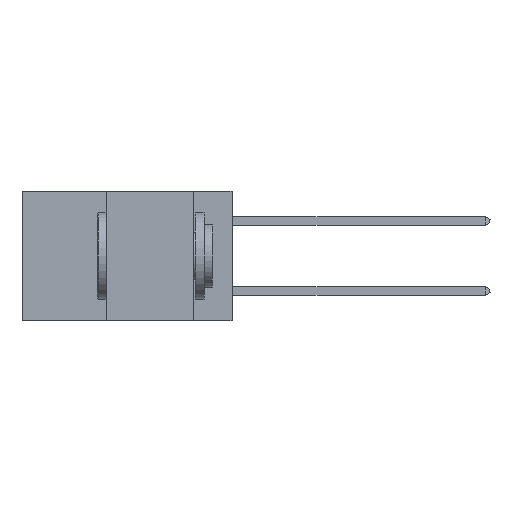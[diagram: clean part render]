
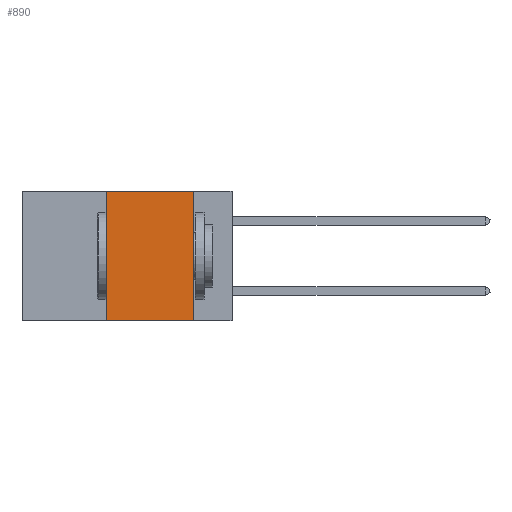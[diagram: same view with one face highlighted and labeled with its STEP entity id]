
A CAD part, left-side view. The second image highlights one B-rep face of the part: STEP entity #890.
In plain terms, the highlighted planar face has unit normal (-1, 0, 0).
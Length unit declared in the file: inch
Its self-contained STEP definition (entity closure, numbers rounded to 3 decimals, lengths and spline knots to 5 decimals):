
#78 = CARTESIAN_POINT ( 'NONE',  ( 0., 0.36, -0.37 ) ) ;
#890 = ADVANCED_FACE ( 'NONE', ( #15110 ), #18830, .F. ) ;
#2411 = EDGE_CURVE ( 'NONE', #33484, #6966, #22947, .T. ) ;
#3220 = ORIENTED_EDGE ( 'NONE', *, *, #2411, .F. ) ;
#4472 = DIRECTION ( 'NONE',  ( 0., 0., -1. ) ) ;
#5048 = VECTOR ( 'NONE', #7545, 39.37008 ) ;
#5586 = ORIENTED_EDGE ( 'NONE', *, *, #13845, .F. ) ;
#6966 = VERTEX_POINT ( 'NONE', #10816 ) ;
#7545 = DIRECTION ( 'NONE',  ( 0., 0., 1. ) ) ;
#10816 = CARTESIAN_POINT ( 'NONE',  ( 0., 0.36, 0. ) ) ;
#13380 = VECTOR ( 'NONE', #4472, 39.37008 ) ;
#13675 = DIRECTION ( 'NONE',  ( 1., 0., 0. ) ) ;
#13845 = EDGE_CURVE ( 'NONE', #6966, #30428, #28025, .T. ) ;
#15110 = FACE_OUTER_BOUND ( 'NONE', #24315, .T. ) ;
#15184 = LINE ( 'NONE', #33421, #28493 ) ;
#15223 = CARTESIAN_POINT ( 'NONE',  ( 0., 0.36, 0. ) ) ;
#15521 = CARTESIAN_POINT ( 'NONE',  ( 0., 0.11, 0. ) ) ;
#17452 = EDGE_CURVE ( 'NONE', #33484, #20964, #15184, .T. ) ;
#18069 = CARTESIAN_POINT ( 'NONE',  ( 0., 0.11, -0.37 ) ) ;
#18830 = PLANE ( 'NONE',  #19981 ) ;
#19981 = AXIS2_PLACEMENT_3D ( 'NONE', #29602, #13675, #32253 ) ;
#19999 = DIRECTION ( 'NONE',  ( 0., -1., 0. ) ) ;
#20700 = ORIENTED_EDGE ( 'NONE', *, *, #31818, .F. ) ;
#20918 = CARTESIAN_POINT ( 'NONE',  ( 0., 0.11, 0. ) ) ;
#20964 = VERTEX_POINT ( 'NONE', #18069 ) ;
#21262 = ORIENTED_EDGE ( 'NONE', *, *, #17452, .T. ) ;
#22947 = LINE ( 'NONE', #15223, #5048 ) ;
#24315 = EDGE_LOOP ( 'NONE', ( #20700, #5586, #3220, #21262 ) ) ;
#25784 = CARTESIAN_POINT ( 'NONE',  ( 0., 0.6, 0. ) ) ;
#28025 = LINE ( 'NONE', #25784, #29258 ) ;
#28429 = DIRECTION ( 'NONE',  ( 0., -1., 0. ) ) ;
#28493 = VECTOR ( 'NONE', #19999, 39.37008 ) ;
#29185 = LINE ( 'NONE', #20918, #13380 ) ;
#29258 = VECTOR ( 'NONE', #28429, 39.37008 ) ;
#29602 = CARTESIAN_POINT ( 'NONE',  ( 0., 0.6, 0. ) ) ;
#30428 = VERTEX_POINT ( 'NONE', #15521 ) ;
#31818 = EDGE_CURVE ( 'NONE', #30428, #20964, #29185, .T. ) ;
#32253 = DIRECTION ( 'NONE',  ( 0., 0., -1. ) ) ;
#33421 = CARTESIAN_POINT ( 'NONE',  ( 0., 0.6, -0.37 ) ) ;
#33484 = VERTEX_POINT ( 'NONE', #78 ) ;
